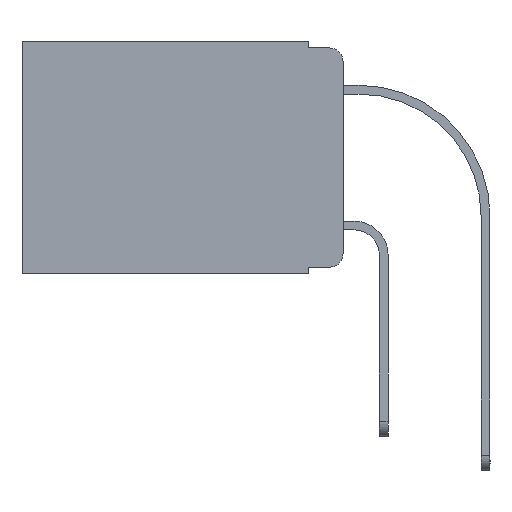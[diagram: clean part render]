
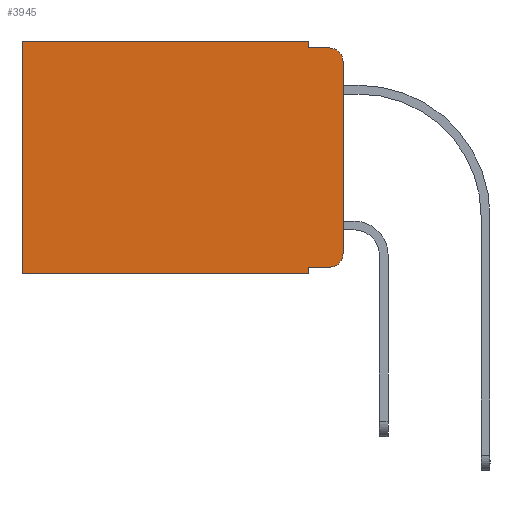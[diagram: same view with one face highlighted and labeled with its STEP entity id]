
A CAD part, left-side view. The second image highlights one B-rep face of the part: STEP entity #3945.
In plain terms, the highlighted planar face has unit normal (-1, 0, 0).
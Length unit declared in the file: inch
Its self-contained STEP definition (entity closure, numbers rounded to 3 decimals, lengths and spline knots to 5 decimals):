
#24 = LINE ( 'NONE', #8162, #11481 ) ;
#499 = DIRECTION ( 'NONE',  ( 0., 0., -1. ) ) ;
#689 = VECTOR ( 'NONE', #6869, 39.37008 ) ;
#707 = ORIENTED_EDGE ( 'NONE', *, *, #6019, .F. ) ;
#928 = PLANE ( 'NONE',  #2014 ) ;
#947 = CARTESIAN_POINT ( 'NONE',  ( 0.298, 0.051, 0. ) ) ;
#1000 = CARTESIAN_POINT ( 'NONE',  ( 0.298, 0., 0. ) ) ;
#1160 = ORIENTED_EDGE ( 'NONE', *, *, #3506, .F. ) ;
#1268 = VERTEX_POINT ( 'NONE', #9716 ) ;
#1422 = CIRCLE ( 'NONE', #7017, 0.02 ) ;
#1621 = VERTEX_POINT ( 'NONE', #8171 ) ;
#2014 = AXIS2_PLACEMENT_3D ( 'NONE', #1000, #7002, #4222 ) ;
#2145 = VERTEX_POINT ( 'NONE', #11560 ) ;
#2210 = DIRECTION ( 'NONE',  ( 0., 0., -1. ) ) ;
#2791 = ORIENTED_EDGE ( 'NONE', *, *, #3530, .T. ) ;
#2916 = CARTESIAN_POINT ( 'NONE',  ( 0.298, 0., -0.03 ) ) ;
#3379 = CARTESIAN_POINT ( 'NONE',  ( 0.298, 0.02, -0.313 ) ) ;
#3380 = CARTESIAN_POINT ( 'NONE',  ( 0.298, 0.473, 0. ) ) ;
#3506 = EDGE_CURVE ( 'NONE', #8363, #12893, #10155, .T. ) ;
#3530 = EDGE_CURVE ( 'NONE', #3934, #1268, #1422, .T. ) ;
#3567 = LINE ( 'NONE', #7730, #689 ) ;
#3683 = CARTESIAN_POINT ( 'NONE',  ( 0.298, 0.02, -0.03 ) ) ;
#3758 = VECTOR ( 'NONE', #12442, 39.37008 ) ;
#3934 = VERTEX_POINT ( 'NONE', #10213 ) ;
#3945 = ADVANCED_FACE ( 'NONE', ( #7069 ), #928, .F. ) ;
#4222 = DIRECTION ( 'NONE',  ( 0., 0., -1. ) ) ;
#4259 = LINE ( 'NONE', #7563, #3758 ) ;
#4562 = EDGE_CURVE ( 'NONE', #8363, #3934, #8914, .T. ) ;
#4838 = CARTESIAN_POINT ( 'NONE',  ( 0.298, 0.051, -0.333 ) ) ;
#4936 = LINE ( 'NONE', #8109, #6986 ) ;
#4939 = ORIENTED_EDGE ( 'NONE', *, *, #10090, .T. ) ;
#5333 = ORIENTED_EDGE ( 'NONE', *, *, #12108, .F. ) ;
#5583 = DIRECTION ( 'NONE',  ( -1., 0., 0. ) ) ;
#5693 = AXIS2_PLACEMENT_3D ( 'NONE', #3683, #7723, #5709 ) ;
#5709 = DIRECTION ( 'NONE',  ( 0., 0., -1. ) ) ;
#5880 = EDGE_CURVE ( 'NONE', #10728, #1268, #11717, .T. ) ;
#6019 = EDGE_CURVE ( 'NONE', #2145, #1621, #4936, .T. ) ;
#6027 = ORIENTED_EDGE ( 'NONE', *, *, #5880, .F. ) ;
#6118 = EDGE_CURVE ( 'NONE', #11544, #6934, #4259, .T. ) ;
#6150 = DIRECTION ( 'NONE',  ( 0., 0., -1. ) ) ;
#6612 = CARTESIAN_POINT ( 'NONE',  ( 0.298, 0.473, -0.343 ) ) ;
#6792 = CARTESIAN_POINT ( 'NONE',  ( 0.298, 0.051, -0.343 ) ) ;
#6869 = DIRECTION ( 'NONE',  ( 0., 1., 0. ) ) ;
#6934 = VERTEX_POINT ( 'NONE', #3380 ) ;
#6986 = VECTOR ( 'NONE', #13256, 39.37008 ) ;
#7002 = DIRECTION ( 'NONE',  ( 1., 0., 0. ) ) ;
#7017 = AXIS2_PLACEMENT_3D ( 'NONE', #3379, #5583, #8677 ) ;
#7030 = EDGE_CURVE ( 'NONE', #12893, #8253, #3567, .T. ) ;
#7069 = FACE_OUTER_BOUND ( 'NONE', #8397, .T. ) ;
#7337 = LINE ( 'NONE', #10615, #11887 ) ;
#7563 = CARTESIAN_POINT ( 'NONE',  ( 0.298, 0., 0. ) ) ;
#7723 = DIRECTION ( 'NONE',  ( -1., 0., 0. ) ) ;
#7730 = CARTESIAN_POINT ( 'NONE',  ( 0.298, 0., -0.343 ) ) ;
#7744 = ORIENTED_EDGE ( 'NONE', *, *, #6118, .T. ) ;
#7772 = CARTESIAN_POINT ( 'NONE',  ( 0.298, 0.051, 0. ) ) ;
#8109 = CARTESIAN_POINT ( 'NONE',  ( 0.298, 0.051, -0.01 ) ) ;
#8162 = CARTESIAN_POINT ( 'NONE',  ( 0.298, 0.051, 0. ) ) ;
#8171 = CARTESIAN_POINT ( 'NONE',  ( 0.298, 0.02, -0.01 ) ) ;
#8253 = VERTEX_POINT ( 'NONE', #6612 ) ;
#8363 = VERTEX_POINT ( 'NONE', #4838 ) ;
#8397 = EDGE_LOOP ( 'NONE', ( #6027, #4939, #707, #5333, #7744, #8688, #10259, #1160, #9571, #2791 ) ) ;
#8474 = VECTOR ( 'NONE', #11973, 39.37008 ) ;
#8644 = CARTESIAN_POINT ( 'NONE',  ( 0.298, 0.051, -0.333 ) ) ;
#8677 = DIRECTION ( 'NONE',  ( 0., 0., -1. ) ) ;
#8688 = ORIENTED_EDGE ( 'NONE', *, *, #11389, .T. ) ;
#8717 = CARTESIAN_POINT ( 'NONE',  ( 0.298, 0., 0. ) ) ;
#8914 = LINE ( 'NONE', #8644, #8474 ) ;
#9571 = ORIENTED_EDGE ( 'NONE', *, *, #4562, .T. ) ;
#9716 = CARTESIAN_POINT ( 'NONE',  ( 0.298, 0., -0.313 ) ) ;
#10090 = EDGE_CURVE ( 'NONE', #10728, #1621, #11691, .T. ) ;
#10155 = LINE ( 'NONE', #947, #11707 ) ;
#10213 = CARTESIAN_POINT ( 'NONE',  ( 0.298, 0.02, -0.333 ) ) ;
#10259 = ORIENTED_EDGE ( 'NONE', *, *, #7030, .F. ) ;
#10615 = CARTESIAN_POINT ( 'NONE',  ( 0.298, 0.473, 0. ) ) ;
#10728 = VERTEX_POINT ( 'NONE', #2916 ) ;
#10818 = VECTOR ( 'NONE', #499, 39.37008 ) ;
#11389 = EDGE_CURVE ( 'NONE', #6934, #8253, #7337, .T. ) ;
#11481 = VECTOR ( 'NONE', #6150, 39.37008 ) ;
#11544 = VERTEX_POINT ( 'NONE', #7772 ) ;
#11560 = CARTESIAN_POINT ( 'NONE',  ( 0.298, 0.051, -0.01 ) ) ;
#11691 = CIRCLE ( 'NONE', #5693, 0.02 ) ;
#11707 = VECTOR ( 'NONE', #13235, 39.37008 ) ;
#11717 = LINE ( 'NONE', #8717, #10818 ) ;
#11887 = VECTOR ( 'NONE', #2210, 39.37008 ) ;
#11973 = DIRECTION ( 'NONE',  ( 0., -1., 0. ) ) ;
#12108 = EDGE_CURVE ( 'NONE', #11544, #2145, #24, .T. ) ;
#12442 = DIRECTION ( 'NONE',  ( 0., 1., 0. ) ) ;
#12893 = VERTEX_POINT ( 'NONE', #6792 ) ;
#13235 = DIRECTION ( 'NONE',  ( 0., 0., -1. ) ) ;
#13256 = DIRECTION ( 'NONE',  ( 0., -1., 0. ) ) ;
